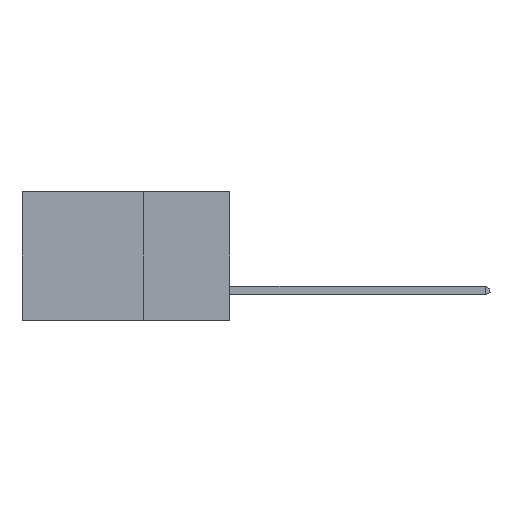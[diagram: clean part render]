
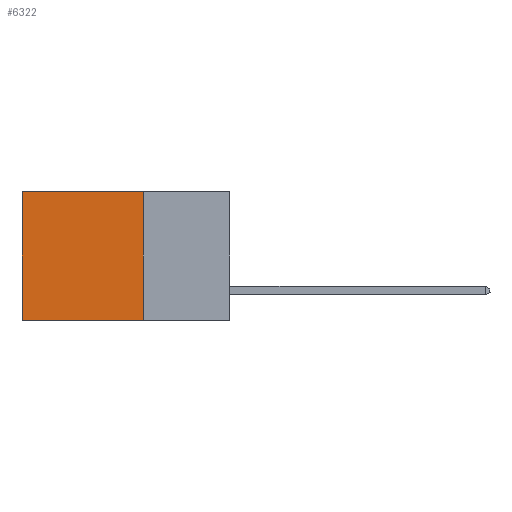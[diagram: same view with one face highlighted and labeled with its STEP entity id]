
A CAD part, left-side view. The second image highlights one B-rep face of the part: STEP entity #6322.
In plain terms, the highlighted planar face has unit normal (-1, 0, 0).
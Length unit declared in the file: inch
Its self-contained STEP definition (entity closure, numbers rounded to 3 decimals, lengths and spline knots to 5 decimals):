
#189 = VERTEX_POINT ( 'NONE', #2384 ) ;
#208 = ORIENTED_EDGE ( 'NONE', *, *, #3927, .F. ) ;
#1140 = DIRECTION ( 'NONE',  ( 0., 0., -1. ) ) ;
#1471 = FACE_OUTER_BOUND ( 'NONE', #6715, .T. ) ;
#1549 = LINE ( 'NONE', #6661, #2193 ) ;
#1824 = DIRECTION ( 'NONE',  ( 0., 0., -1. ) ) ;
#1906 = CARTESIAN_POINT ( 'NONE',  ( 0.298, 0.6, -0.37 ) ) ;
#2193 = VECTOR ( 'NONE', #9206, 39.37008 ) ;
#2224 = VECTOR ( 'NONE', #7058, 39.37008 ) ;
#2384 = CARTESIAN_POINT ( 'NONE',  ( 0.298, 0.25, 0. ) ) ;
#2834 = CARTESIAN_POINT ( 'NONE',  ( 0.298, 0.25, -0.37 ) ) ;
#3395 = EDGE_CURVE ( 'NONE', #6892, #10654, #5765, .T. ) ;
#3927 = EDGE_CURVE ( 'NONE', #189, #6892, #8364, .T. ) ;
#4197 = ORIENTED_EDGE ( 'NONE', *, *, #3395, .F. ) ;
#4594 = CARTESIAN_POINT ( 'NONE',  ( 0.298, 0.6, 0. ) ) ;
#5154 = ORIENTED_EDGE ( 'NONE', *, *, #7571, .T. ) ;
#5765 = LINE ( 'NONE', #2834, #9412 ) ;
#5968 = ORIENTED_EDGE ( 'NONE', *, *, #8943, .T. ) ;
#6174 = CARTESIAN_POINT ( 'NONE',  ( 0.298, 0.25, 0. ) ) ;
#6322 = ADVANCED_FACE ( 'NONE', ( #1471 ), #10331, .F. ) ;
#6479 = AXIS2_PLACEMENT_3D ( 'NONE', #6174, #10400, #1140 ) ;
#6661 = CARTESIAN_POINT ( 'NONE',  ( 0.298, 0.25, 0. ) ) ;
#6715 = EDGE_LOOP ( 'NONE', ( #5154, #4197, #208, #5968 ) ) ;
#6835 = CARTESIAN_POINT ( 'NONE',  ( 0.298, 0.25, 0. ) ) ;
#6892 = VERTEX_POINT ( 'NONE', #7051 ) ;
#7051 = CARTESIAN_POINT ( 'NONE',  ( 0.298, 0.25, -0.37 ) ) ;
#7058 = DIRECTION ( 'NONE',  ( 0., 0., -1. ) ) ;
#7571 = EDGE_CURVE ( 'NONE', #9232, #10654, #10725, .T. ) ;
#7837 = VECTOR ( 'NONE', #1824, 39.37008 ) ;
#8364 = LINE ( 'NONE', #6835, #7837 ) ;
#8943 = EDGE_CURVE ( 'NONE', #189, #9232, #1549, .T. ) ;
#9165 = CARTESIAN_POINT ( 'NONE',  ( 0.298, 0.6, 0. ) ) ;
#9206 = DIRECTION ( 'NONE',  ( 0., 1., 0. ) ) ;
#9232 = VERTEX_POINT ( 'NONE', #9165 ) ;
#9412 = VECTOR ( 'NONE', #10375, 39.37008 ) ;
#10331 = PLANE ( 'NONE',  #6479 ) ;
#10375 = DIRECTION ( 'NONE',  ( 0., 1., 0. ) ) ;
#10400 = DIRECTION ( 'NONE',  ( 1., 0., 0. ) ) ;
#10654 = VERTEX_POINT ( 'NONE', #1906 ) ;
#10725 = LINE ( 'NONE', #4594, #2224 ) ;
